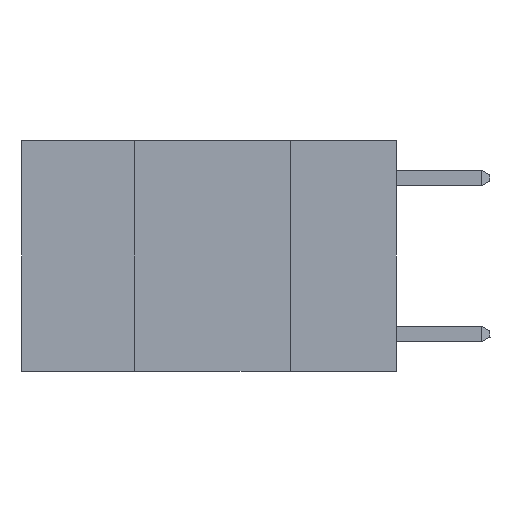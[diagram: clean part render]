
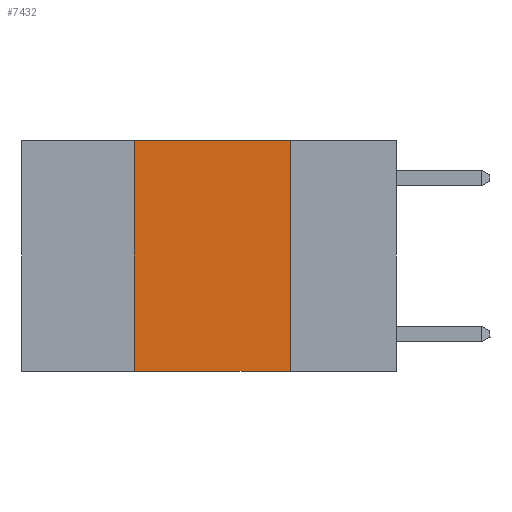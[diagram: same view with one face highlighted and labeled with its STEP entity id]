
A CAD part, left-side view. The second image highlights one B-rep face of the part: STEP entity #7432.
In plain terms, the highlighted planar face has unit normal (-1, 0, 0).
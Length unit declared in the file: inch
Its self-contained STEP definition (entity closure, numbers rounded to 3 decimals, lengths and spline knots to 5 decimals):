
#190 = PLANE ( 'NONE',  #5645 ) ;
#514 = DIRECTION ( 'NONE',  ( 0., -1., 0. ) ) ;
#1221 = DIRECTION ( 'NONE',  ( 0., 0., -1. ) ) ;
#1231 = VECTOR ( 'NONE', #514, 39.37008 ) ;
#1256 = ORIENTED_EDGE ( 'NONE', *, *, #11332, .F. ) ;
#1534 = EDGE_LOOP ( 'NONE', ( #1256, #6506, #3241, #6274 ) ) ;
#1974 = VECTOR ( 'NONE', #3575, 39.37008 ) ;
#2468 = CARTESIAN_POINT ( 'NONE',  ( 0., 0.6, -0.37 ) ) ;
#2615 = CARTESIAN_POINT ( 'NONE',  ( 0., 0.42, 0. ) ) ;
#3154 = VECTOR ( 'NONE', #3707, 39.37008 ) ;
#3241 = ORIENTED_EDGE ( 'NONE', *, *, #11487, .F. ) ;
#3428 = FACE_OUTER_BOUND ( 'NONE', #1534, .T. ) ;
#3575 = DIRECTION ( 'NONE',  ( 0., -1., 0. ) ) ;
#3707 = DIRECTION ( 'NONE',  ( 0., 0., 1. ) ) ;
#4088 = LINE ( 'NONE', #12637, #1231 ) ;
#5218 = LINE ( 'NONE', #2468, #1974 ) ;
#5476 = CARTESIAN_POINT ( 'NONE',  ( 0., 0.6, 0. ) ) ;
#5645 = AXIS2_PLACEMENT_3D ( 'NONE', #5476, #7491, #1221 ) ;
#6160 = LINE ( 'NONE', #12416, #8525 ) ;
#6231 = CARTESIAN_POINT ( 'NONE',  ( 0., 0.17, 0. ) ) ;
#6274 = ORIENTED_EDGE ( 'NONE', *, *, #11414, .T. ) ;
#6506 = ORIENTED_EDGE ( 'NONE', *, *, #8292, .F. ) ;
#6811 = CARTESIAN_POINT ( 'NONE',  ( 0., 0.42, 0. ) ) ;
#6992 = CARTESIAN_POINT ( 'NONE',  ( 0., 0.17, -0.37 ) ) ;
#7432 = ADVANCED_FACE ( 'NONE', ( #3428 ), #190, .F. ) ;
#7491 = DIRECTION ( 'NONE',  ( 1., 0., 0. ) ) ;
#8292 = EDGE_CURVE ( 'NONE', #11451, #9474, #4088, .T. ) ;
#8525 = VECTOR ( 'NONE', #8582, 39.37008 ) ;
#8582 = DIRECTION ( 'NONE',  ( 0., 0., -1. ) ) ;
#9474 = VERTEX_POINT ( 'NONE', #6231 ) ;
#10571 = VERTEX_POINT ( 'NONE', #6992 ) ;
#11250 = LINE ( 'NONE', #2615, #3154 ) ;
#11332 = EDGE_CURVE ( 'NONE', #9474, #10571, #6160, .T. ) ;
#11414 = EDGE_CURVE ( 'NONE', #11784, #10571, #5218, .T. ) ;
#11451 = VERTEX_POINT ( 'NONE', #6811 ) ;
#11487 = EDGE_CURVE ( 'NONE', #11784, #11451, #11250, .T. ) ;
#11784 = VERTEX_POINT ( 'NONE', #12873 ) ;
#12416 = CARTESIAN_POINT ( 'NONE',  ( 0., 0.17, 0. ) ) ;
#12637 = CARTESIAN_POINT ( 'NONE',  ( 0., 0.6, 0. ) ) ;
#12873 = CARTESIAN_POINT ( 'NONE',  ( 0., 0.42, -0.37 ) ) ;
